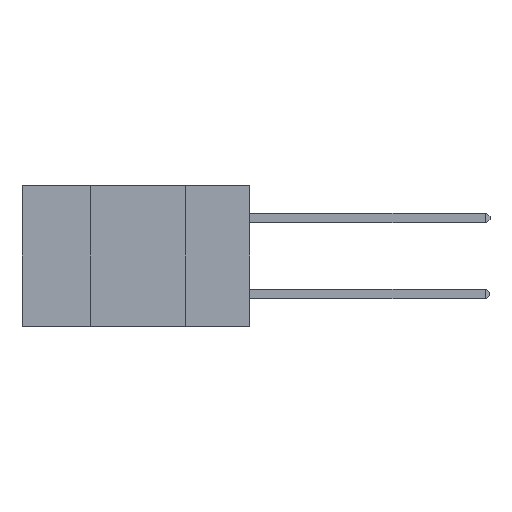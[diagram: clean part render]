
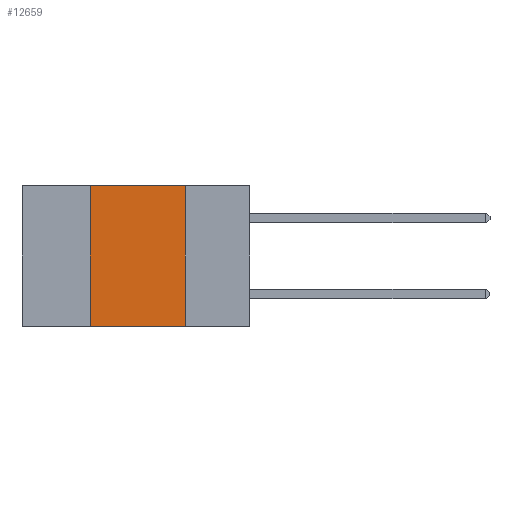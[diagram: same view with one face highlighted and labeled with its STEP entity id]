
A CAD part, left-side view. The second image highlights one B-rep face of the part: STEP entity #12659.
In plain terms, the highlighted planar face has unit normal (-1, 0, 0).
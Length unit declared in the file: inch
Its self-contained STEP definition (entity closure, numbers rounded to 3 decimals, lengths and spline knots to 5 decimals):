
#3 = DIRECTION ( 'NONE',  ( 0., -1., 0. ) ) ;
#404 = EDGE_CURVE ( 'NONE', #7617, #1604, #4656, .T. ) ;
#1116 = LINE ( 'NONE', #4777, #4262 ) ;
#1597 = VECTOR ( 'NONE', #3, 39.37008 ) ;
#1604 = VERTEX_POINT ( 'NONE', #3669 ) ;
#2994 = VERTEX_POINT ( 'NONE', #3248 ) ;
#3223 = CARTESIAN_POINT ( 'NONE',  ( 0., 0.42, 0. ) ) ;
#3248 = CARTESIAN_POINT ( 'NONE',  ( 0., 0.17, -0.37 ) ) ;
#3545 = DIRECTION ( 'NONE',  ( 0., 0., -1. ) ) ;
#3669 = CARTESIAN_POINT ( 'NONE',  ( 0., 0.17, 0. ) ) ;
#3695 = CARTESIAN_POINT ( 'NONE',  ( 0., 0.42, -0.37 ) ) ;
#3711 = DIRECTION ( 'NONE',  ( 0., -1., 0. ) ) ;
#4262 = VECTOR ( 'NONE', #3545, 39.37008 ) ;
#4656 = LINE ( 'NONE', #8612, #14799 ) ;
#4704 = CARTESIAN_POINT ( 'NONE',  ( 0., 0.6, 0. ) ) ;
#4777 = CARTESIAN_POINT ( 'NONE',  ( 0., 0.17, 0. ) ) ;
#5204 = AXIS2_PLACEMENT_3D ( 'NONE', #4704, #14515, #7192 ) ;
#5341 = FACE_OUTER_BOUND ( 'NONE', #9816, .T. ) ;
#5560 = ORIENTED_EDGE ( 'NONE', *, *, #11439, .F. ) ;
#5637 = ORIENTED_EDGE ( 'NONE', *, *, #404, .F. ) ;
#6531 = CARTESIAN_POINT ( 'NONE',  ( 0., 0.6, -0.37 ) ) ;
#7192 = DIRECTION ( 'NONE',  ( 0., 0., -1. ) ) ;
#7617 = VERTEX_POINT ( 'NONE', #3223 ) ;
#8612 = CARTESIAN_POINT ( 'NONE',  ( 0., 0.6, 0. ) ) ;
#9202 = LINE ( 'NONE', #6531, #1597 ) ;
#9706 = PLANE ( 'NONE',  #5204 ) ;
#9777 = LINE ( 'NONE', #14606, #15756 ) ;
#9816 = EDGE_LOOP ( 'NONE', ( #5560, #5637, #14191, #12672 ) ) ;
#11439 = EDGE_CURVE ( 'NONE', #1604, #2994, #1116, .T. ) ;
#12157 = VERTEX_POINT ( 'NONE', #3695 ) ;
#12659 = ADVANCED_FACE ( 'NONE', ( #5341 ), #9706, .F. ) ;
#12672 = ORIENTED_EDGE ( 'NONE', *, *, #15006, .T. ) ;
#14191 = ORIENTED_EDGE ( 'NONE', *, *, #14734, .F. ) ;
#14515 = DIRECTION ( 'NONE',  ( 1., 0., 0. ) ) ;
#14606 = CARTESIAN_POINT ( 'NONE',  ( 0., 0.42, 0. ) ) ;
#14734 = EDGE_CURVE ( 'NONE', #12157, #7617, #9777, .T. ) ;
#14799 = VECTOR ( 'NONE', #3711, 39.37008 ) ;
#15006 = EDGE_CURVE ( 'NONE', #12157, #2994, #9202, .T. ) ;
#15756 = VECTOR ( 'NONE', #15800, 39.37008 ) ;
#15800 = DIRECTION ( 'NONE',  ( 0., 0., 1. ) ) ;
